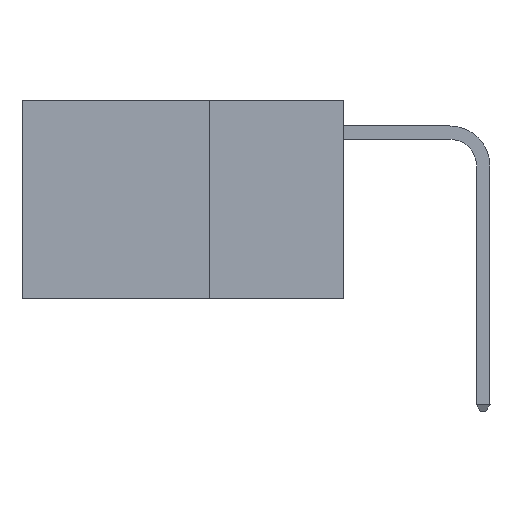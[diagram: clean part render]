
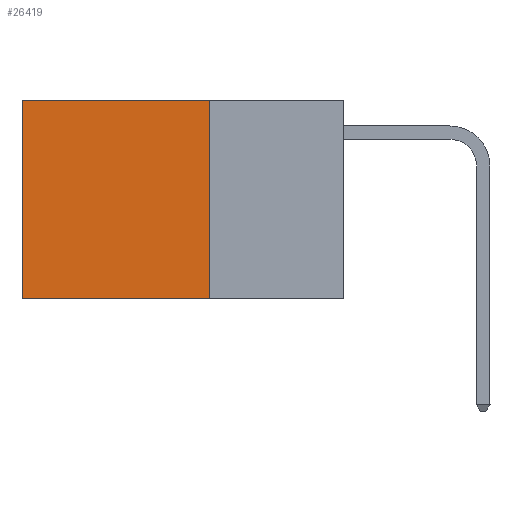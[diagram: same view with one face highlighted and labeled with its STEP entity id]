
A CAD part, left-side view. The second image highlights one B-rep face of the part: STEP entity #26419.
In plain terms, the highlighted planar face has unit normal (-1, 0, 0).
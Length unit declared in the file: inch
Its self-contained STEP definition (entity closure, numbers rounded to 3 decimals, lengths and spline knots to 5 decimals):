
#271 = CARTESIAN_POINT ( 'NONE',  ( 0.2625, 0.25, 0. ) ) ;
#603 = ORIENTED_EDGE ( 'NONE', *, *, #16551, .F. ) ;
#1726 = LINE ( 'NONE', #21319, #13551 ) ;
#2676 = DIRECTION ( 'NONE',  ( 0., 1., 0. ) ) ;
#3108 = ORIENTED_EDGE ( 'NONE', *, *, #21550, .T. ) ;
#4512 = AXIS2_PLACEMENT_3D ( 'NONE', #9315, #11718, #27583 ) ;
#5351 = VERTEX_POINT ( 'NONE', #27320 ) ;
#7804 = LINE ( 'NONE', #22490, #20151 ) ;
#8670 = DIRECTION ( 'NONE',  ( 0., 0., -1. ) ) ;
#8873 = DIRECTION ( 'NONE',  ( 0., 1., 0. ) ) ;
#9036 = CARTESIAN_POINT ( 'NONE',  ( 0.2625, 0.6, 0. ) ) ;
#9315 = CARTESIAN_POINT ( 'NONE',  ( 0.2625, 0.25, 0. ) ) ;
#9732 = FACE_OUTER_BOUND ( 'NONE', #18554, .T. ) ;
#9856 = CARTESIAN_POINT ( 'NONE',  ( 0.2625, 0.25, 0. ) ) ;
#11718 = DIRECTION ( 'NONE',  ( 1., 0., 0. ) ) ;
#13551 = VECTOR ( 'NONE', #23591, 39.37008 ) ;
#13676 = VERTEX_POINT ( 'NONE', #15995 ) ;
#15995 = CARTESIAN_POINT ( 'NONE',  ( 0.2625, 0.6, -0.37 ) ) ;
#16489 = EDGE_CURVE ( 'NONE', #27690, #13676, #7804, .T. ) ;
#16551 = EDGE_CURVE ( 'NONE', #5351, #13676, #18763, .T. ) ;
#18065 = VECTOR ( 'NONE', #8873, 39.37008 ) ;
#18554 = EDGE_LOOP ( 'NONE', ( #29642, #603, #25826, #3108 ) ) ;
#18763 = LINE ( 'NONE', #20440, #18065 ) ;
#20151 = VECTOR ( 'NONE', #8670, 39.37008 ) ;
#20440 = CARTESIAN_POINT ( 'NONE',  ( 0.2625, 0.25, -0.37 ) ) ;
#21319 = CARTESIAN_POINT ( 'NONE',  ( 0.2625, 0.25, 0. ) ) ;
#21550 = EDGE_CURVE ( 'NONE', #26583, #27690, #28388, .T. ) ;
#22468 = VECTOR ( 'NONE', #2676, 39.37008 ) ;
#22490 = CARTESIAN_POINT ( 'NONE',  ( 0.2625, 0.6, 0. ) ) ;
#22760 = EDGE_CURVE ( 'NONE', #26583, #5351, #1726, .T. ) ;
#23115 = PLANE ( 'NONE',  #4512 ) ;
#23591 = DIRECTION ( 'NONE',  ( 0., 0., -1. ) ) ;
#25826 = ORIENTED_EDGE ( 'NONE', *, *, #22760, .F. ) ;
#26419 = ADVANCED_FACE ( 'NONE', ( #9732 ), #23115, .F. ) ;
#26583 = VERTEX_POINT ( 'NONE', #9856 ) ;
#27320 = CARTESIAN_POINT ( 'NONE',  ( 0.2625, 0.25, -0.37 ) ) ;
#27583 = DIRECTION ( 'NONE',  ( 0., 0., -1. ) ) ;
#27690 = VERTEX_POINT ( 'NONE', #9036 ) ;
#28388 = LINE ( 'NONE', #271, #22468 ) ;
#29642 = ORIENTED_EDGE ( 'NONE', *, *, #16489, .T. ) ;
